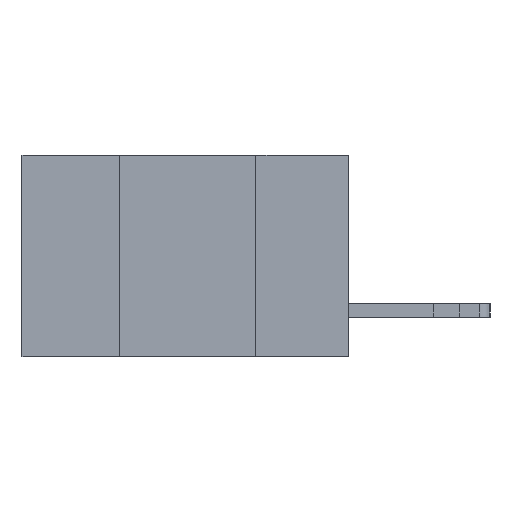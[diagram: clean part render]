
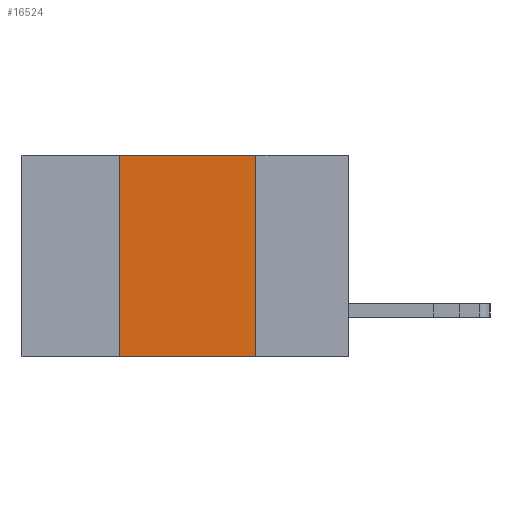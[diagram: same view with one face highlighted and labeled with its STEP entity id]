
A CAD part, left-side view. The second image highlights one B-rep face of the part: STEP entity #16524.
In plain terms, the highlighted planar face has unit normal (-1, 0, 0).
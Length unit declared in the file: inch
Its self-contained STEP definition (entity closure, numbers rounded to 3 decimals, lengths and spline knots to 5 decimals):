
#556 = VECTOR ( 'NONE', #673, 39.37008 ) ;
#575 = DIRECTION ( 'NONE',  ( 0., 0., -1. ) ) ;
#673 = DIRECTION ( 'NONE',  ( 0., -1., 0. ) ) ;
#754 = CARTESIAN_POINT ( 'NONE',  ( 0., 0.6, -0.37 ) ) ;
#1303 = CARTESIAN_POINT ( 'NONE',  ( 0., 0.17, -0.37 ) ) ;
#1490 = ORIENTED_EDGE ( 'NONE', *, *, #3666, .T. ) ;
#2203 = VECTOR ( 'NONE', #575, 39.37008 ) ;
#2637 = LINE ( 'NONE', #17552, #2203 ) ;
#3142 = VECTOR ( 'NONE', #11362, 39.37008 ) ;
#3269 = VERTEX_POINT ( 'NONE', #10169 ) ;
#3666 = EDGE_CURVE ( 'NONE', #15918, #8518, #16106, .T. ) ;
#4810 = CARTESIAN_POINT ( 'NONE',  ( 0., 0.42, -0.37 ) ) ;
#5912 = PLANE ( 'NONE',  #14149 ) ;
#6536 = EDGE_CURVE ( 'NONE', #15918, #3269, #6934, .T. ) ;
#6934 = LINE ( 'NONE', #14282, #3142 ) ;
#7314 = DIRECTION ( 'NONE',  ( 0., 0., -1. ) ) ;
#7621 = EDGE_CURVE ( 'NONE', #3269, #18343, #17912, .T. ) ;
#7718 = ORIENTED_EDGE ( 'NONE', *, *, #9380, .F. ) ;
#8518 = VERTEX_POINT ( 'NONE', #1303 ) ;
#9380 = EDGE_CURVE ( 'NONE', #18343, #8518, #2637, .T. ) ;
#10169 = CARTESIAN_POINT ( 'NONE',  ( 0., 0.42, 0. ) ) ;
#10211 = FACE_OUTER_BOUND ( 'NONE', #13195, .T. ) ;
#10433 = VECTOR ( 'NONE', #13583, 39.37008 ) ;
#11362 = DIRECTION ( 'NONE',  ( 0., 0., 1. ) ) ;
#11538 = CARTESIAN_POINT ( 'NONE',  ( 0., 0.17, 0. ) ) ;
#12173 = CARTESIAN_POINT ( 'NONE',  ( 0., 0.6, 0. ) ) ;
#12610 = ORIENTED_EDGE ( 'NONE', *, *, #6536, .F. ) ;
#13049 = ORIENTED_EDGE ( 'NONE', *, *, #7621, .F. ) ;
#13195 = EDGE_LOOP ( 'NONE', ( #7718, #13049, #12610, #1490 ) ) ;
#13583 = DIRECTION ( 'NONE',  ( 0., -1., 0. ) ) ;
#14149 = AXIS2_PLACEMENT_3D ( 'NONE', #14316, #15775, #7314 ) ;
#14282 = CARTESIAN_POINT ( 'NONE',  ( 0., 0.42, 0. ) ) ;
#14316 = CARTESIAN_POINT ( 'NONE',  ( 0., 0.6, 0. ) ) ;
#15775 = DIRECTION ( 'NONE',  ( 1., 0., 0. ) ) ;
#15918 = VERTEX_POINT ( 'NONE', #4810 ) ;
#16106 = LINE ( 'NONE', #754, #556 ) ;
#16524 = ADVANCED_FACE ( 'NONE', ( #10211 ), #5912, .F. ) ;
#17552 = CARTESIAN_POINT ( 'NONE',  ( 0., 0.17, 0. ) ) ;
#17912 = LINE ( 'NONE', #12173, #10433 ) ;
#18343 = VERTEX_POINT ( 'NONE', #11538 ) ;
